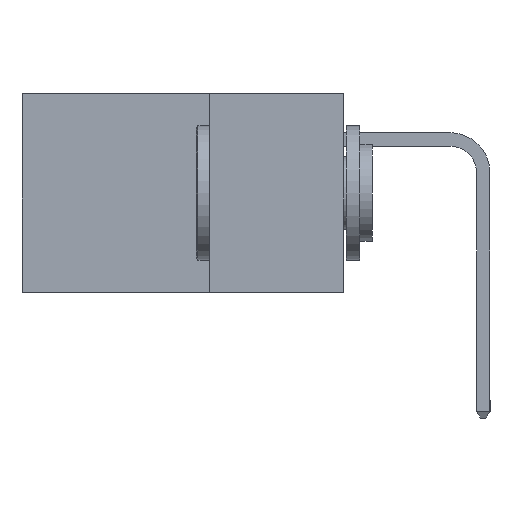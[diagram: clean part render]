
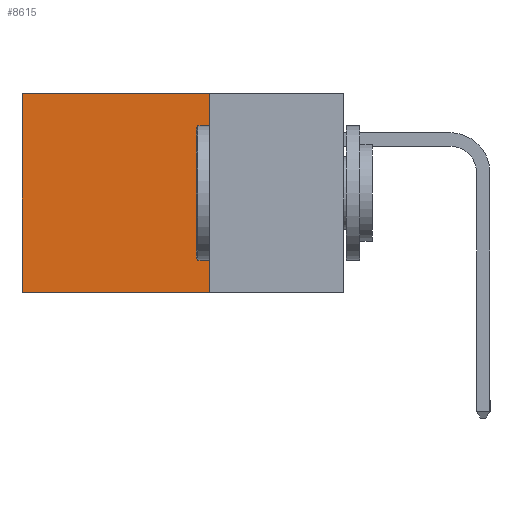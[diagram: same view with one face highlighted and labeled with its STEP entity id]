
A CAD part, left-side view. The second image highlights one B-rep face of the part: STEP entity #8615.
In plain terms, the highlighted planar face has unit normal (-1, 0, 0).
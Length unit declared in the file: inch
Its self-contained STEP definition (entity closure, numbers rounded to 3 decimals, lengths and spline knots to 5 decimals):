
#265 = CARTESIAN_POINT ( 'NONE',  ( 0.2615, 0.25, -0.37 ) ) ;
#519 = VERTEX_POINT ( 'NONE', #12324 ) ;
#2090 = LINE ( 'NONE', #16624, #5723 ) ;
#3264 = CARTESIAN_POINT ( 'NONE',  ( 0.2615, 0.25, -0.37 ) ) ;
#3574 = ORIENTED_EDGE ( 'NONE', *, *, #10279, .F. ) ;
#4026 = VECTOR ( 'NONE', #14254, 39.37008 ) ;
#4311 = DIRECTION ( 'NONE',  ( 0., 1., 0. ) ) ;
#5170 = ORIENTED_EDGE ( 'NONE', *, *, #14862, .F. ) ;
#5723 = VECTOR ( 'NONE', #4311, 39.37008 ) ;
#5961 = VECTOR ( 'NONE', #17247, 39.37008 ) ;
#6555 = VERTEX_POINT ( 'NONE', #7777 ) ;
#6599 = ORIENTED_EDGE ( 'NONE', *, *, #12568, .T. ) ;
#7610 = CARTESIAN_POINT ( 'NONE',  ( 0.2615, 0.6, 0. ) ) ;
#7777 = CARTESIAN_POINT ( 'NONE',  ( 0.2615, 0.25, 0. ) ) ;
#8319 = VECTOR ( 'NONE', #11666, 39.37008 ) ;
#8615 = ADVANCED_FACE ( 'NONE', ( #9342 ), #18589, .F. ) ;
#8702 = EDGE_LOOP ( 'NONE', ( #6599, #3574, #5170, #16702 ) ) ;
#9004 = AXIS2_PLACEMENT_3D ( 'NONE', #18178, #18039, #17935 ) ;
#9342 = FACE_OUTER_BOUND ( 'NONE', #8702, .T. ) ;
#9921 = VERTEX_POINT ( 'NONE', #3264 ) ;
#10108 = LINE ( 'NONE', #15773, #5961 ) ;
#10279 = EDGE_CURVE ( 'NONE', #9921, #519, #12740, .T. ) ;
#11666 = DIRECTION ( 'NONE',  ( 0., 0., -1. ) ) ;
#12324 = CARTESIAN_POINT ( 'NONE',  ( 0.2615, 0.6, -0.37 ) ) ;
#12363 = EDGE_CURVE ( 'NONE', #6555, #16280, #2090, .T. ) ;
#12435 = LINE ( 'NONE', #13201, #8319 ) ;
#12568 = EDGE_CURVE ( 'NONE', #16280, #519, #10108, .T. ) ;
#12740 = LINE ( 'NONE', #265, #4026 ) ;
#13201 = CARTESIAN_POINT ( 'NONE',  ( 0.2615, 0.25, -0.37 ) ) ;
#14254 = DIRECTION ( 'NONE',  ( 0., 1., 0. ) ) ;
#14862 = EDGE_CURVE ( 'NONE', #6555, #9921, #12435, .T. ) ;
#15773 = CARTESIAN_POINT ( 'NONE',  ( 0.2615, 0.6, -0.37 ) ) ;
#16280 = VERTEX_POINT ( 'NONE', #7610 ) ;
#16624 = CARTESIAN_POINT ( 'NONE',  ( 0.2615, 0.25, 0. ) ) ;
#16702 = ORIENTED_EDGE ( 'NONE', *, *, #12363, .T. ) ;
#17247 = DIRECTION ( 'NONE',  ( 0., 0., -1. ) ) ;
#17935 = DIRECTION ( 'NONE',  ( 0., 0., -1. ) ) ;
#18039 = DIRECTION ( 'NONE',  ( 1., 0., 0. ) ) ;
#18178 = CARTESIAN_POINT ( 'NONE',  ( 0.2615, 0.25, -0.37 ) ) ;
#18589 = PLANE ( 'NONE',  #9004 ) ;
